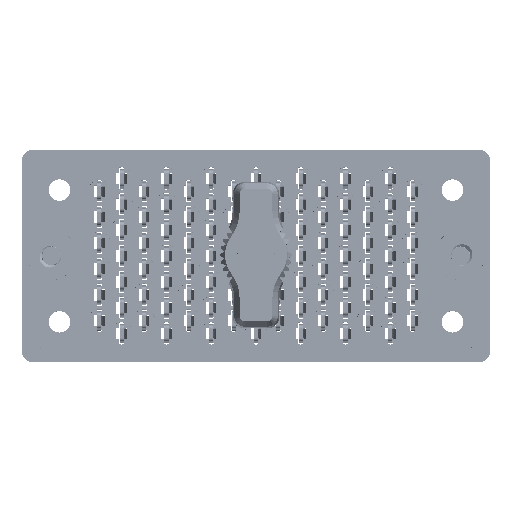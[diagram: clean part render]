
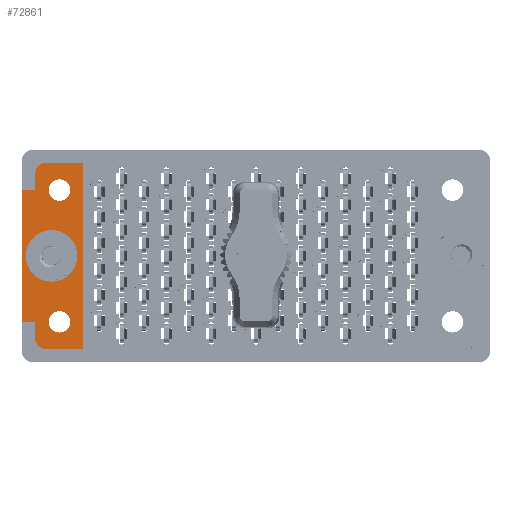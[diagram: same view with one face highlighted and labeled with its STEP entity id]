
A CAD part, top view. The second image highlights one B-rep face of the part: STEP entity #72861.
In plain terms, the highlighted planar face has unit normal (0, 0, 1).
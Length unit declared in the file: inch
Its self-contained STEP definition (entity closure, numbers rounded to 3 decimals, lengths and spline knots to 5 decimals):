
#204 = PLANE ( 'NONE',  #60509 ) ;
#242 = DIRECTION ( 'NONE',  ( 0., 0., 1. ) ) ;
#658 = DIRECTION ( 'NONE',  ( 1., 0., 0. ) ) ;
#741 = EDGE_CURVE ( 'NONE', #70355, #29684, #93310, .T. ) ;
#1176 = FACE_BOUND ( 'NONE', #91560, .T. ) ;
#1954 = VECTOR ( 'NONE', #92321, 39.37008 ) ;
#2278 = LINE ( 'NONE', #25233, #3706 ) ;
#3456 = DIRECTION ( 'NONE',  ( 0., 0., 1. ) ) ;
#3463 = EDGE_CURVE ( 'NONE', #71778, #10682, #20312, .T. ) ;
#3566 = CIRCLE ( 'NONE', #86369, 0.062 ) ;
#3706 = VECTOR ( 'NONE', #76118, 39.37008 ) ;
#4789 = EDGE_CURVE ( 'NONE', #35593, #70355, #24957, .T. ) ;
#4982 = DIRECTION ( 'NONE',  ( 0., 0., 1. ) ) ;
#6354 = VERTEX_POINT ( 'NONE', #11750 ) ;
#6528 = DIRECTION ( 'NONE',  ( 1., 0., 0. ) ) ;
#7126 = EDGE_CURVE ( 'NONE', #78328, #11464, #67494, .T. ) ;
#7386 = EDGE_CURVE ( 'NONE', #90396, #75053, #64386, .T. ) ;
#8027 = DIRECTION ( 'NONE',  ( 0., 0., 1. ) ) ;
#8370 = CARTESIAN_POINT ( 'NONE',  ( -1.0785, -0.3825, -0.117 ) ) ;
#8445 = CARTESIAN_POINT ( 'NONE',  ( -1.2825, 0.3825, -0.117 ) ) ;
#8984 = FACE_OUTER_BOUND ( 'NONE', #66985, .T. ) ;
#10682 = VERTEX_POINT ( 'NONE', #46208 ) ;
#11464 = VERTEX_POINT ( 'NONE', #46814 ) ;
#11615 = EDGE_CURVE ( 'NONE', #10682, #71778, #21031, .T. ) ;
#11750 = CARTESIAN_POINT ( 'NONE',  ( -1.3375, 0., -0.117 ) ) ;
#13770 = VECTOR ( 'NONE', #35149, 39.37008 ) ;
#13870 = DIRECTION ( 'NONE',  ( 0., 0., 1. ) ) ;
#13998 = CARTESIAN_POINT ( 'NONE',  ( -1.005, -0.54, -0.117 ) ) ;
#15425 = CARTESIAN_POINT ( 'NONE',  ( -1.0785, 0.3825, -0.117 ) ) ;
#17606 = VECTOR ( 'NONE', #69096, 39.37008 ) ;
#17654 = CARTESIAN_POINT ( 'NONE',  ( -1.1875, 0., -0.117 ) ) ;
#17751 = CIRCLE ( 'NONE', #88060, 0.0625 ) ;
#18131 = DIRECTION ( 'NONE',  ( 1., 0., 0. ) ) ;
#20312 = CIRCLE ( 'NONE', #57809, 0.0625 ) ;
#21031 = CIRCLE ( 'NONE', #89783, 0.0625 ) ;
#21177 = CARTESIAN_POINT ( 'NONE',  ( -1.141, -0.3825, -0.117 ) ) ;
#21415 = CARTESIAN_POINT ( 'NONE',  ( -1.359, 0.3825, -0.117 ) ) ;
#21737 = VERTEX_POINT ( 'NONE', #15425 ) ;
#23378 = ORIENTED_EDGE ( 'NONE', *, *, #7126, .T. ) ;
#24957 = LINE ( 'NONE', #77284, #65820 ) ;
#25012 = EDGE_CURVE ( 'NONE', #58101, #75053, #73013, .T. ) ;
#25129 = VERTEX_POINT ( 'NONE', #8445 ) ;
#25233 = CARTESIAN_POINT ( 'NONE',  ( 0., -0.54, -0.117 ) ) ;
#25337 = AXIS2_PLACEMENT_3D ( 'NONE', #42623, #4982, #94947 ) ;
#25340 = CARTESIAN_POINT ( 'NONE',  ( 0., 0.54, -0.117 ) ) ;
#25669 = LINE ( 'NONE', #63787, #63709 ) ;
#25723 = VERTEX_POINT ( 'NONE', #78556 ) ;
#27326 = CARTESIAN_POINT ( 'NONE',  ( -1.141, 0.3825, -0.117 ) ) ;
#27554 = DIRECTION ( 'NONE',  ( -1., 0., 0. ) ) ;
#28457 = ORIENTED_EDGE ( 'NONE', *, *, #39770, .T. ) ;
#29684 = VERTEX_POINT ( 'NONE', #39275 ) ;
#30632 = CARTESIAN_POINT ( 'NONE',  ( -1.359, -0.3825, -0.117 ) ) ;
#31446 = CARTESIAN_POINT ( 'NONE',  ( -1.141, -0.3825, -0.117 ) ) ;
#34528 = EDGE_CURVE ( 'NONE', #56661, #6354, #77061, .T. ) ;
#35149 = DIRECTION ( 'NONE',  ( -1., 0., 0. ) ) ;
#35388 = CARTESIAN_POINT ( 'NONE',  ( -1.2205, 0.478, -0.117 ) ) ;
#35593 = VERTEX_POINT ( 'NONE', #13998 ) ;
#36480 = VECTOR ( 'NONE', #27554, 39.37008 ) ;
#36846 = CARTESIAN_POINT ( 'NONE',  ( -1.0375, 0., -0.117 ) ) ;
#36864 = CARTESIAN_POINT ( 'NONE',  ( -1.141, 0.3825, -0.117 ) ) ;
#39275 = CARTESIAN_POINT ( 'NONE',  ( -1.2205, 0.54, -0.117 ) ) ;
#39770 = EDGE_CURVE ( 'NONE', #58101, #78328, #25669, .T. ) ;
#40787 = CIRCLE ( 'NONE', #87647, 0.0625 ) ;
#41730 = ORIENTED_EDGE ( 'NONE', *, *, #4789, .T. ) ;
#41863 = EDGE_CURVE ( 'NONE', #6354, #56661, #84285, .T. ) ;
#42503 = LINE ( 'NONE', #72331, #13770 ) ;
#42623 = CARTESIAN_POINT ( 'NONE',  ( -1.2205, -0.478, -0.117 ) ) ;
#44204 = DIRECTION ( 'NONE',  ( 0., 0., 1. ) ) ;
#45429 = EDGE_CURVE ( 'NONE', #47810, #25129, #91628, .T. ) ;
#46208 = CARTESIAN_POINT ( 'NONE',  ( -1.2035, -0.3825, -0.117 ) ) ;
#46814 = CARTESIAN_POINT ( 'NONE',  ( -1.2205, -0.54, -0.117 ) ) ;
#47810 = VERTEX_POINT ( 'NONE', #94340 ) ;
#48329 = ORIENTED_EDGE ( 'NONE', *, *, #85698, .T. ) ;
#48858 = DIRECTION ( 'NONE',  ( 1., 0., 0. ) ) ;
#49841 = EDGE_LOOP ( 'NONE', ( #54510, #59136 ) ) ;
#50297 = DIRECTION ( 'NONE',  ( 0., 0., 1. ) ) ;
#51160 = ORIENTED_EDGE ( 'NONE', *, *, #3463, .F. ) ;
#51970 = CARTESIAN_POINT ( 'NONE',  ( 0., -0.3825, -0.117 ) ) ;
#52255 = CARTESIAN_POINT ( 'NONE',  ( -1.2825, -0.3825, -0.117 ) ) ;
#53489 = CARTESIAN_POINT ( 'NONE',  ( -1.2825, 0., -0.117 ) ) ;
#53842 = DIRECTION ( 'NONE',  ( 0., 1., 0. ) ) ;
#54478 = ORIENTED_EDGE ( 'NONE', *, *, #96307, .F. ) ;
#54510 = ORIENTED_EDGE ( 'NONE', *, *, #34528, .F. ) ;
#56129 = DIRECTION ( 'NONE',  ( -1., 0., 0. ) ) ;
#56141 = AXIS2_PLACEMENT_3D ( 'NONE', #17654, #3456, #18131 ) ;
#56275 = EDGE_CURVE ( 'NONE', #25129, #90396, #42503, .T. ) ;
#56661 = VERTEX_POINT ( 'NONE', #36846 ) ;
#57809 = AXIS2_PLACEMENT_3D ( 'NONE', #31446, #61274, #658 ) ;
#58101 = VERTEX_POINT ( 'NONE', #52255 ) ;
#58187 = EDGE_LOOP ( 'NONE', ( #76937, #89886 ) ) ;
#58829 = DIRECTION ( 'NONE',  ( 0., 0., 1. ) ) ;
#59136 = ORIENTED_EDGE ( 'NONE', *, *, #41863, .F. ) ;
#60137 = EDGE_CURVE ( 'NONE', #21737, #25723, #40787, .T. ) ;
#60509 = AXIS2_PLACEMENT_3D ( 'NONE', #75029, #8027, #90688 ) ;
#60648 = VECTOR ( 'NONE', #56129, 39.37008 ) ;
#61274 = DIRECTION ( 'NONE',  ( 0., 0., 1. ) ) ;
#61314 = FACE_BOUND ( 'NONE', #49841, .T. ) ;
#63709 = VECTOR ( 'NONE', #77496, 39.37008 ) ;
#63787 = CARTESIAN_POINT ( 'NONE',  ( -1.2825, 0., -0.117 ) ) ;
#64252 = CARTESIAN_POINT ( 'NONE',  ( -1.005, 0.54, -0.117 ) ) ;
#64386 = LINE ( 'NONE', #85941, #1954 ) ;
#65807 = CARTESIAN_POINT ( 'NONE',  ( -1.2825, -0.478, -0.117 ) ) ;
#65820 = VECTOR ( 'NONE', #53842, 39.37008 ) ;
#66265 = CARTESIAN_POINT ( 'NONE',  ( -1.1875, 0., -0.117 ) ) ;
#66985 = EDGE_LOOP ( 'NONE', ( #28457, #23378, #54478, #41730, #74608, #48329, #84963, #78157, #83370, #88937 ) ) ;
#67196 = FACE_BOUND ( 'NONE', #58187, .T. ) ;
#67494 = CIRCLE ( 'NONE', #25337, 0.062 ) ;
#69096 = DIRECTION ( 'NONE',  ( 0., -1., 0. ) ) ;
#70355 = VERTEX_POINT ( 'NONE', #64252 ) ;
#71708 = DIRECTION ( 'NONE',  ( 1., 0., 0. ) ) ;
#71778 = VERTEX_POINT ( 'NONE', #8370 ) ;
#72331 = CARTESIAN_POINT ( 'NONE',  ( 0., 0.3825, -0.117 ) ) ;
#72387 = AXIS2_PLACEMENT_3D ( 'NONE', #66265, #242, #74083 ) ;
#72861 = ADVANCED_FACE ( 'NONE', ( #1176, #67196, #61314, #8984 ), #204, .T. ) ;
#73013 = LINE ( 'NONE', #51970, #36480 ) ;
#74083 = DIRECTION ( 'NONE',  ( 1., 0., 0. ) ) ;
#74608 = ORIENTED_EDGE ( 'NONE', *, *, #741, .T. ) ;
#75029 = CARTESIAN_POINT ( 'NONE',  ( -1.359, -0.617, -0.117 ) ) ;
#75053 = VERTEX_POINT ( 'NONE', #30632 ) ;
#76118 = DIRECTION ( 'NONE',  ( -1., 0., 0. ) ) ;
#76937 = ORIENTED_EDGE ( 'NONE', *, *, #84655, .F. ) ;
#77061 = CIRCLE ( 'NONE', #72387, 0.15 ) ;
#77284 = CARTESIAN_POINT ( 'NONE',  ( -1.005, 0.617, -0.117 ) ) ;
#77496 = DIRECTION ( 'NONE',  ( 0., -1., 0. ) ) ;
#78157 = ORIENTED_EDGE ( 'NONE', *, *, #56275, .T. ) ;
#78328 = VERTEX_POINT ( 'NONE', #65807 ) ;
#78556 = CARTESIAN_POINT ( 'NONE',  ( -1.2035, 0.3825, -0.117 ) ) ;
#79273 = ORIENTED_EDGE ( 'NONE', *, *, #11615, .F. ) ;
#83370 = ORIENTED_EDGE ( 'NONE', *, *, #7386, .T. ) ;
#84285 = CIRCLE ( 'NONE', #56141, 0.15 ) ;
#84655 = EDGE_CURVE ( 'NONE', #25723, #21737, #17751, .T. ) ;
#84963 = ORIENTED_EDGE ( 'NONE', *, *, #45429, .T. ) ;
#85698 = EDGE_CURVE ( 'NONE', #29684, #47810, #3566, .T. ) ;
#85941 = CARTESIAN_POINT ( 'NONE',  ( -1.359, 0.617, -0.117 ) ) ;
#86369 = AXIS2_PLACEMENT_3D ( 'NONE', #35388, #13870, #6528 ) ;
#87647 = AXIS2_PLACEMENT_3D ( 'NONE', #36864, #44204, #94622 ) ;
#88060 = AXIS2_PLACEMENT_3D ( 'NONE', #27326, #50297, #48858 ) ;
#88937 = ORIENTED_EDGE ( 'NONE', *, *, #25012, .F. ) ;
#89783 = AXIS2_PLACEMENT_3D ( 'NONE', #21177, #58829, #71708 ) ;
#89886 = ORIENTED_EDGE ( 'NONE', *, *, #60137, .F. ) ;
#90396 = VERTEX_POINT ( 'NONE', #21415 ) ;
#90688 = DIRECTION ( 'NONE',  ( 1., 0., 0. ) ) ;
#91560 = EDGE_LOOP ( 'NONE', ( #79273, #51160 ) ) ;
#91628 = LINE ( 'NONE', #53489, #17606 ) ;
#92321 = DIRECTION ( 'NONE',  ( 0., -1., 0. ) ) ;
#93310 = LINE ( 'NONE', #25340, #60648 ) ;
#94340 = CARTESIAN_POINT ( 'NONE',  ( -1.2825, 0.478, -0.117 ) ) ;
#94622 = DIRECTION ( 'NONE',  ( 1., 0., 0. ) ) ;
#94947 = DIRECTION ( 'NONE',  ( 1., 0., 0. ) ) ;
#96307 = EDGE_CURVE ( 'NONE', #35593, #11464, #2278, .T. ) ;
